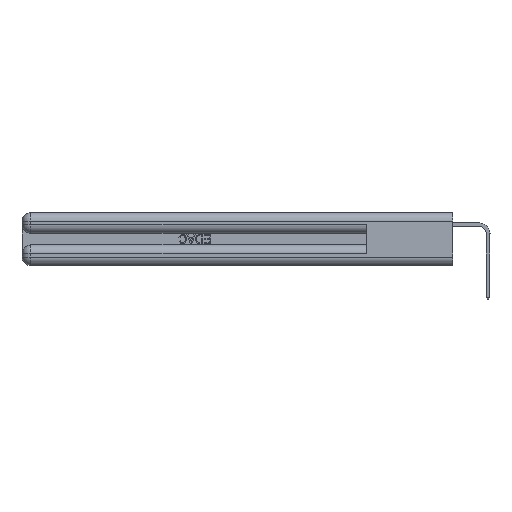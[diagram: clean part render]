
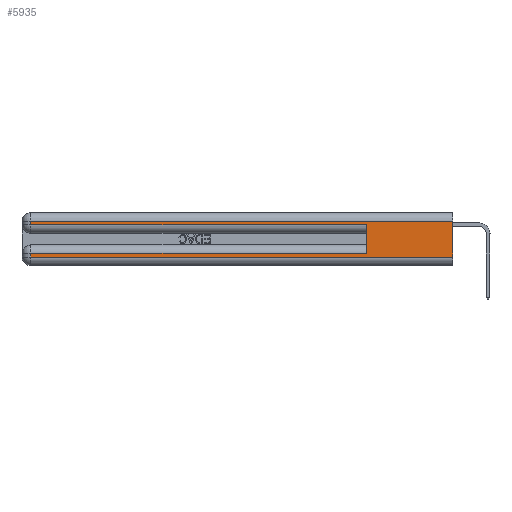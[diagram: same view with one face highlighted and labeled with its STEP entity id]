
A CAD part, left-side view. The second image highlights one B-rep face of the part: STEP entity #5935.
In plain terms, the highlighted planar face has unit normal (-1, 0, 0).
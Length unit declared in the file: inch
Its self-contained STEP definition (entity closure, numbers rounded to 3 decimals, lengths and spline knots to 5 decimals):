
#1659 = ORIENTED_EDGE ( 'NONE', *, *, #47972, .F. ) ;
#2247 = VECTOR ( 'NONE', #54337, 39.37008 ) ;
#3178 = CARTESIAN_POINT ( 'NONE',  ( 0., 0., 0.31 ) ) ;
#3872 = ORIENTED_EDGE ( 'NONE', *, *, #45365, .T. ) ;
#4109 = CARTESIAN_POINT ( 'NONE',  ( 0., 2.94, 0.06 ) ) ;
#4847 = VERTEX_POINT ( 'NONE', #29178 ) ;
#4987 = CARTESIAN_POINT ( 'NONE',  ( 0., 2.94, 0.085 ) ) ;
#5483 = CARTESIAN_POINT ( 'NONE',  ( 0., 2.94, 0.37 ) ) ;
#5618 = CARTESIAN_POINT ( 'NONE',  ( 0., 0.6, 0.085 ) ) ;
#5935 = ADVANCED_FACE ( 'NONE', ( #41705 ), #6670, .F. ) ;
#6536 = CARTESIAN_POINT ( 'NONE',  ( 0., 2.94, 0.31 ) ) ;
#6663 = LINE ( 'NONE', #10147, #16668 ) ;
#6670 = PLANE ( 'NONE',  #51610 ) ;
#7413 = VECTOR ( 'NONE', #49877, 39.37008 ) ;
#7451 = DIRECTION ( 'NONE',  ( 0., 1., 0. ) ) ;
#8267 = CARTESIAN_POINT ( 'NONE',  ( 0., 0.6, 0.285 ) ) ;
#9599 = CARTESIAN_POINT ( 'NONE',  ( 0., 0., 0.085 ) ) ;
#9708 = VERTEX_POINT ( 'NONE', #6536 ) ;
#9825 = CARTESIAN_POINT ( 'NONE',  ( 0., 2.94, 0.37 ) ) ;
#10147 = CARTESIAN_POINT ( 'NONE',  ( 0., 0., 0.37 ) ) ;
#11151 = VECTOR ( 'NONE', #39743, 39.37008 ) ;
#11327 = CARTESIAN_POINT ( 'NONE',  ( 0., 0.6, 0.145 ) ) ;
#11875 = ORIENTED_EDGE ( 'NONE', *, *, #25958, .T. ) ;
#14093 = DIRECTION ( 'NONE',  ( 0., 0., -1. ) ) ;
#15256 = EDGE_CURVE ( 'NONE', #48396, #48150, #20105, .T. ) ;
#15258 = DIRECTION ( 'NONE',  ( 1., 0., 0. ) ) ;
#15381 = VERTEX_POINT ( 'NONE', #20636 ) ;
#16668 = VECTOR ( 'NONE', #48503, 39.37008 ) ;
#17957 = VERTEX_POINT ( 'NONE', #4987 ) ;
#18396 = VECTOR ( 'NONE', #49836, 39.37008 ) ;
#20105 = LINE ( 'NONE', #11327, #7413 ) ;
#20317 = EDGE_CURVE ( 'NONE', #9708, #21934, #55338, .T. ) ;
#20636 = CARTESIAN_POINT ( 'NONE',  ( 0., 0., 0.06 ) ) ;
#20687 = LINE ( 'NONE', #9599, #30706 ) ;
#21434 = ORIENTED_EDGE ( 'NONE', *, *, #43331, .T. ) ;
#21934 = VERTEX_POINT ( 'NONE', #33079 ) ;
#22061 = VERTEX_POINT ( 'NONE', #4109 ) ;
#22628 = VECTOR ( 'NONE', #14093, 39.37008 ) ;
#23665 = CARTESIAN_POINT ( 'NONE',  ( 0., 0., 0.37 ) ) ;
#25958 = EDGE_CURVE ( 'NONE', #17957, #22061, #36337, .T. ) ;
#28512 = LINE ( 'NONE', #3178, #49966 ) ;
#29162 = ORIENTED_EDGE ( 'NONE', *, *, #15256, .F. ) ;
#29178 = CARTESIAN_POINT ( 'NONE',  ( 0., 0., 0.31 ) ) ;
#30706 = VECTOR ( 'NONE', #43863, 39.37008 ) ;
#32384 = CARTESIAN_POINT ( 'NONE',  ( 0., 0., 0.285 ) ) ;
#33079 = CARTESIAN_POINT ( 'NONE',  ( 0., 2.94, 0.285 ) ) ;
#35408 = EDGE_LOOP ( 'NONE', ( #1659, #21434, #41643, #55155, #29162, #54633, #11875, #3872 ) ) ;
#36324 = LINE ( 'NONE', #41448, #2247 ) ;
#36337 = LINE ( 'NONE', #9825, #22628 ) ;
#39743 = DIRECTION ( 'NONE',  ( 0., 0., -1. ) ) ;
#41225 = LINE ( 'NONE', #32384, #18396 ) ;
#41448 = CARTESIAN_POINT ( 'NONE',  ( 0., 0., 0.06 ) ) ;
#41643 = ORIENTED_EDGE ( 'NONE', *, *, #20317, .T. ) ;
#41705 = FACE_OUTER_BOUND ( 'NONE', #35408, .T. ) ;
#43331 = EDGE_CURVE ( 'NONE', #4847, #9708, #28512, .T. ) ;
#43863 = DIRECTION ( 'NONE',  ( 0., 1., 0. ) ) ;
#45229 = DIRECTION ( 'NONE',  ( 0., 0., -1. ) ) ;
#45365 = EDGE_CURVE ( 'NONE', #22061, #15381, #36324, .T. ) ;
#47897 = EDGE_CURVE ( 'NONE', #48396, #17957, #20687, .T. ) ;
#47972 = EDGE_CURVE ( 'NONE', #4847, #15381, #6663, .T. ) ;
#48150 = VERTEX_POINT ( 'NONE', #8267 ) ;
#48396 = VERTEX_POINT ( 'NONE', #5618 ) ;
#48503 = DIRECTION ( 'NONE',  ( 0., 0., -1. ) ) ;
#49836 = DIRECTION ( 'NONE',  ( 0., -1., 0. ) ) ;
#49877 = DIRECTION ( 'NONE',  ( 0., 0., 1. ) ) ;
#49966 = VECTOR ( 'NONE', #7451, 39.37008 ) ;
#51145 = EDGE_CURVE ( 'NONE', #21934, #48150, #41225, .T. ) ;
#51610 = AXIS2_PLACEMENT_3D ( 'NONE', #23665, #15258, #45229 ) ;
#54337 = DIRECTION ( 'NONE',  ( 0., -1., 0. ) ) ;
#54633 = ORIENTED_EDGE ( 'NONE', *, *, #47897, .T. ) ;
#55155 = ORIENTED_EDGE ( 'NONE', *, *, #51145, .T. ) ;
#55338 = LINE ( 'NONE', #5483, #11151 ) ;
